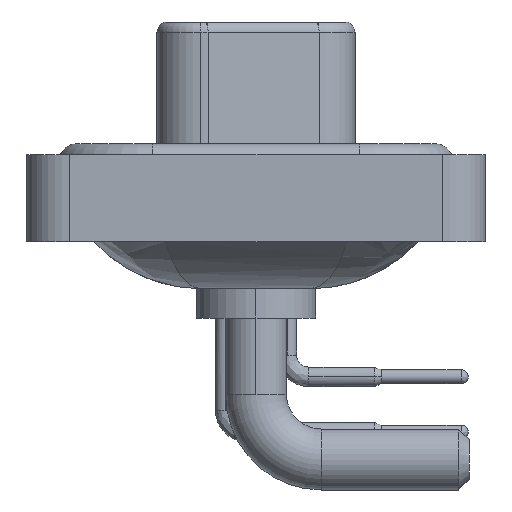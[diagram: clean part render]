
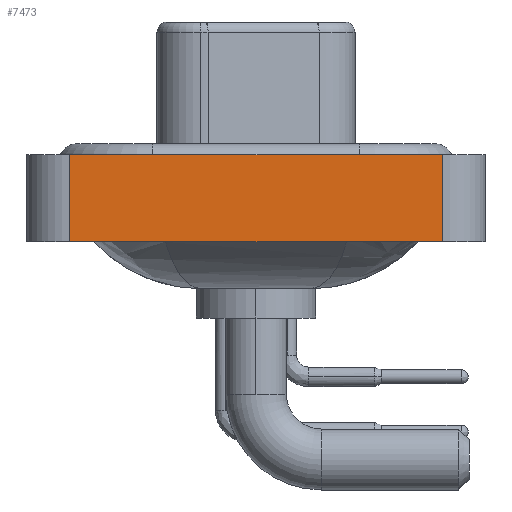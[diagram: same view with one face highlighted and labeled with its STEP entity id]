
A CAD part, left-side view. The second image highlights one B-rep face of the part: STEP entity #7473.
In plain terms, the highlighted planar face has unit normal (-1, 0, 0).
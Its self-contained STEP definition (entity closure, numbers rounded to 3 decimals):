
#201 = EDGE_CURVE ( 'NONE', #16490, #5128, #5254, .T. ) ;
#810 = EDGE_CURVE ( 'NONE', #8201, #14632, #14570, .T. ) ;
#1695 = VECTOR ( 'NONE', #2428, 1000. ) ;
#2233 = DIRECTION ( 'NONE',  ( 0., 0., 1. ) ) ;
#2428 = DIRECTION ( 'NONE',  ( 0., -1., 0. ) ) ;
#3417 = DIRECTION ( 'NONE',  ( 0., -1., 0. ) ) ;
#4468 = DIRECTION ( 'NONE',  ( -1., 0., 0. ) ) ;
#4732 = ORIENTED_EDGE ( 'NONE', *, *, #7637, .T. ) ;
#4996 = CARTESIAN_POINT ( 'NONE',  ( -7.35, -8.55, -3.6 ) ) ;
#5101 = VECTOR ( 'NONE', #7119, 1000. ) ;
#5128 = VERTEX_POINT ( 'NONE', #7151 ) ;
#5254 = LINE ( 'NONE', #23353, #25669 ) ;
#5792 = VECTOR ( 'NONE', #2233, 1000. ) ;
#7058 = CARTESIAN_POINT ( 'NONE',  ( -7.35, -8.55, 0.4 ) ) ;
#7119 = DIRECTION ( 'NONE',  ( 0., 0., 1. ) ) ;
#7151 = CARTESIAN_POINT ( 'NONE',  ( -7.35, -8.55, -3.6 ) ) ;
#7261 = LINE ( 'NONE', #4996, #5101 ) ;
#7473 = ADVANCED_FACE ( 'NONE', ( #8861 ), #22579, .T. ) ;
#7637 = EDGE_CURVE ( 'NONE', #5128, #14632, #7261, .T. ) ;
#8201 = VERTEX_POINT ( 'NONE', #14155 ) ;
#8711 = DIRECTION ( 'NONE',  ( 0., 0., 1. ) ) ;
#8861 = FACE_OUTER_BOUND ( 'NONE', #10618, .T. ) ;
#10022 = LINE ( 'NONE', #20185, #5792 ) ;
#10180 = ORIENTED_EDGE ( 'NONE', *, *, #810, .F. ) ;
#10618 = EDGE_LOOP ( 'NONE', ( #4732, #10180, #15070, #17846 ) ) ;
#10813 = CARTESIAN_POINT ( 'NONE',  ( -7.35, -8.55, -3.6 ) ) ;
#14155 = CARTESIAN_POINT ( 'NONE',  ( -7.35, 8.55, 0.4 ) ) ;
#14570 = LINE ( 'NONE', #24236, #1695 ) ;
#14632 = VERTEX_POINT ( 'NONE', #7058 ) ;
#15070 = ORIENTED_EDGE ( 'NONE', *, *, #20376, .F. ) ;
#16490 = VERTEX_POINT ( 'NONE', #19862 ) ;
#17762 = AXIS2_PLACEMENT_3D ( 'NONE', #10813, #4468, #8711 ) ;
#17846 = ORIENTED_EDGE ( 'NONE', *, *, #201, .T. ) ;
#19862 = CARTESIAN_POINT ( 'NONE',  ( -7.35, 8.55, -3.6 ) ) ;
#20185 = CARTESIAN_POINT ( 'NONE',  ( -7.35, 8.55, -3.6 ) ) ;
#20376 = EDGE_CURVE ( 'NONE', #16490, #8201, #10022, .T. ) ;
#22579 = PLANE ( 'NONE',  #17762 ) ;
#23353 = CARTESIAN_POINT ( 'NONE',  ( -7.35, -8.55, -3.6 ) ) ;
#24236 = CARTESIAN_POINT ( 'NONE',  ( -7.35, -8.55, 0.4 ) ) ;
#25669 = VECTOR ( 'NONE', #3417, 1000. ) ;
